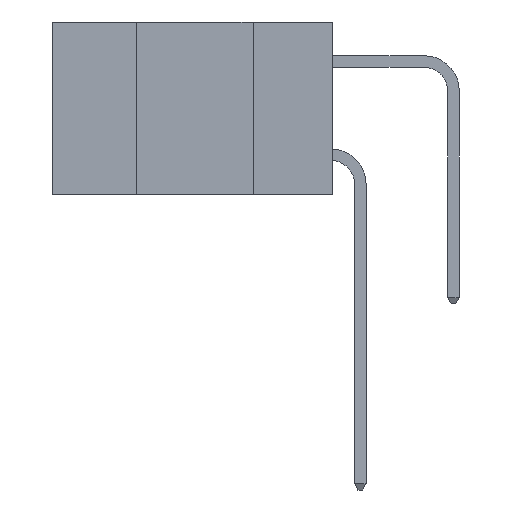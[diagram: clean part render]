
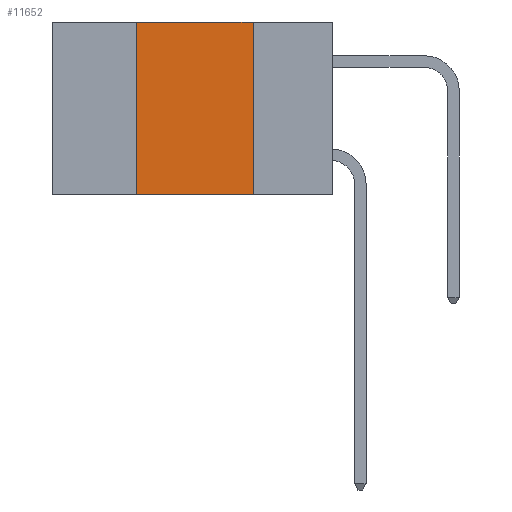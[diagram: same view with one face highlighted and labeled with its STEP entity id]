
A CAD part, left-side view. The second image highlights one B-rep face of the part: STEP entity #11652.
In plain terms, the highlighted planar face has unit normal (-1, 0, 0).
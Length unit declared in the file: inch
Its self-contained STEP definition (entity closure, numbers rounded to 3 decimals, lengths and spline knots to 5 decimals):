
#842 = VERTEX_POINT ( 'NONE', #19643 ) ;
#1000 = LINE ( 'NONE', #7415, #12944 ) ;
#1219 = VERTEX_POINT ( 'NONE', #3656 ) ;
#1245 = EDGE_CURVE ( 'NONE', #18802, #842, #12457, .T. ) ;
#1524 = CARTESIAN_POINT ( 'NONE',  ( 0., 0.42, -0.37 ) ) ;
#2352 = CARTESIAN_POINT ( 'NONE',  ( 0., 0.6, 0. ) ) ;
#2446 = LINE ( 'NONE', #11324, #14352 ) ;
#3117 = DIRECTION ( 'NONE',  ( 0., 0., 1. ) ) ;
#3656 = CARTESIAN_POINT ( 'NONE',  ( 0., 0.42, 0. ) ) ;
#3920 = DIRECTION ( 'NONE',  ( 1., 0., 0. ) ) ;
#4447 = CARTESIAN_POINT ( 'NONE',  ( 0., 0.17, 0. ) ) ;
#4947 = VECTOR ( 'NONE', #3117, 39.37008 ) ;
#5064 = ORIENTED_EDGE ( 'NONE', *, *, #1245, .F. ) ;
#6624 = EDGE_LOOP ( 'NONE', ( #5064, #16438, #12320, #18697 ) ) ;
#7415 = CARTESIAN_POINT ( 'NONE',  ( 0., 0.6, -0.37 ) ) ;
#7607 = DIRECTION ( 'NONE',  ( 0., 0., -1. ) ) ;
#7905 = VERTEX_POINT ( 'NONE', #11442 ) ;
#7913 = EDGE_CURVE ( 'NONE', #1219, #18802, #2446, .T. ) ;
#9059 = AXIS2_PLACEMENT_3D ( 'NONE', #2352, #3920, #14781 ) ;
#9594 = FACE_OUTER_BOUND ( 'NONE', #6624, .T. ) ;
#9923 = CARTESIAN_POINT ( 'NONE',  ( 0., 0.17, -0.37 ) ) ;
#11297 = DIRECTION ( 'NONE',  ( 0., -1., 0. ) ) ;
#11324 = CARTESIAN_POINT ( 'NONE',  ( 0., 0.6, 0. ) ) ;
#11442 = CARTESIAN_POINT ( 'NONE',  ( 0., 0.42, -0.37 ) ) ;
#11652 = ADVANCED_FACE ( 'NONE', ( #9594 ), #17880, .F. ) ;
#12247 = VECTOR ( 'NONE', #7607, 39.37008 ) ;
#12320 = ORIENTED_EDGE ( 'NONE', *, *, #15188, .F. ) ;
#12457 = LINE ( 'NONE', #9923, #12247 ) ;
#12944 = VECTOR ( 'NONE', #19850, 39.37008 ) ;
#13209 = LINE ( 'NONE', #1524, #4947 ) ;
#13229 = EDGE_CURVE ( 'NONE', #7905, #842, #1000, .T. ) ;
#14352 = VECTOR ( 'NONE', #11297, 39.37008 ) ;
#14781 = DIRECTION ( 'NONE',  ( 0., 0., -1. ) ) ;
#15188 = EDGE_CURVE ( 'NONE', #7905, #1219, #13209, .T. ) ;
#16438 = ORIENTED_EDGE ( 'NONE', *, *, #7913, .F. ) ;
#17880 = PLANE ( 'NONE',  #9059 ) ;
#18697 = ORIENTED_EDGE ( 'NONE', *, *, #13229, .T. ) ;
#18802 = VERTEX_POINT ( 'NONE', #4447 ) ;
#19643 = CARTESIAN_POINT ( 'NONE',  ( 0., 0.17, -0.37 ) ) ;
#19850 = DIRECTION ( 'NONE',  ( 0., -1., 0. ) ) ;
